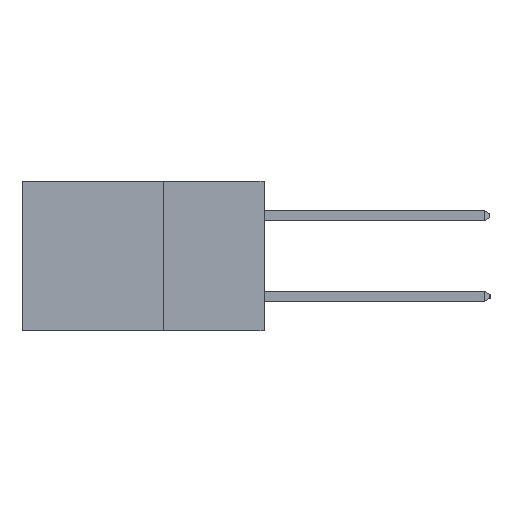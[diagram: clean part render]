
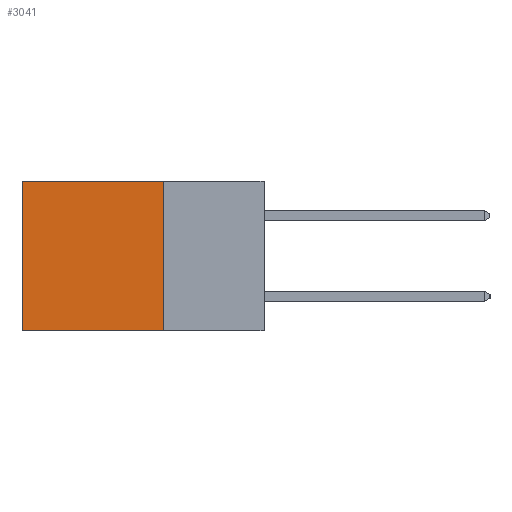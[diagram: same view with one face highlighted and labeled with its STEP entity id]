
A CAD part, left-side view. The second image highlights one B-rep face of the part: STEP entity #3041.
In plain terms, the highlighted planar face has unit normal (-1, 0, 0).
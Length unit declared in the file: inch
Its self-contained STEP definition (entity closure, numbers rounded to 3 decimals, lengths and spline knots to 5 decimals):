
#332 = ORIENTED_EDGE ( 'NONE', *, *, #6425, .F. ) ;
#567 = DIRECTION ( 'NONE',  ( 0., 1., 0. ) ) ;
#807 = CARTESIAN_POINT ( 'NONE',  ( 0.2615, 0.25, 0. ) ) ;
#886 = CARTESIAN_POINT ( 'NONE',  ( 0.2615, 0.25, -0.37 ) ) ;
#1542 = AXIS2_PLACEMENT_3D ( 'NONE', #5706, #8288, #3043 ) ;
#1579 = VERTEX_POINT ( 'NONE', #807 ) ;
#2264 = VERTEX_POINT ( 'NONE', #9968 ) ;
#2341 = VERTEX_POINT ( 'NONE', #3122 ) ;
#3041 = ADVANCED_FACE ( 'NONE', ( #8326 ), #9948, .F. ) ;
#3043 = DIRECTION ( 'NONE',  ( 0., 0., -1. ) ) ;
#3122 = CARTESIAN_POINT ( 'NONE',  ( 0.2615, 0.6, 0. ) ) ;
#3479 = ORIENTED_EDGE ( 'NONE', *, *, #8227, .T. ) ;
#3774 = EDGE_CURVE ( 'NONE', #1579, #10707, #7980, .T. ) ;
#3847 = VECTOR ( 'NONE', #7431, 39.37008 ) ;
#4026 = EDGE_CURVE ( 'NONE', #2341, #2264, #10570, .T. ) ;
#4866 = DIRECTION ( 'NONE',  ( 0., 0., -1. ) ) ;
#5706 = CARTESIAN_POINT ( 'NONE',  ( 0.2615, 0.25, -0.37 ) ) ;
#5800 = VECTOR ( 'NONE', #10179, 39.37008 ) ;
#6425 = EDGE_CURVE ( 'NONE', #10707, #2264, #11121, .T. ) ;
#6559 = CARTESIAN_POINT ( 'NONE',  ( 0.2615, 0.25, 0. ) ) ;
#6810 = CARTESIAN_POINT ( 'NONE',  ( 0.2615, 0.6, -0.37 ) ) ;
#6983 = VECTOR ( 'NONE', #567, 39.37008 ) ;
#7431 = DIRECTION ( 'NONE',  ( 0., 1., 0. ) ) ;
#7980 = LINE ( 'NONE', #886, #10199 ) ;
#8084 = CARTESIAN_POINT ( 'NONE',  ( 0.2615, 0.25, -0.37 ) ) ;
#8227 = EDGE_CURVE ( 'NONE', #1579, #2341, #10627, .T. ) ;
#8288 = DIRECTION ( 'NONE',  ( 1., 0., 0. ) ) ;
#8326 = FACE_OUTER_BOUND ( 'NONE', #10441, .T. ) ;
#9801 = ORIENTED_EDGE ( 'NONE', *, *, #4026, .T. ) ;
#9948 = PLANE ( 'NONE',  #1542 ) ;
#9968 = CARTESIAN_POINT ( 'NONE',  ( 0.2615, 0.6, -0.37 ) ) ;
#10071 = ORIENTED_EDGE ( 'NONE', *, *, #3774, .F. ) ;
#10179 = DIRECTION ( 'NONE',  ( 0., 0., -1. ) ) ;
#10199 = VECTOR ( 'NONE', #4866, 39.37008 ) ;
#10441 = EDGE_LOOP ( 'NONE', ( #9801, #332, #10071, #3479 ) ) ;
#10570 = LINE ( 'NONE', #6810, #5800 ) ;
#10627 = LINE ( 'NONE', #6559, #3847 ) ;
#10707 = VERTEX_POINT ( 'NONE', #8084 ) ;
#11121 = LINE ( 'NONE', #11288, #6983 ) ;
#11288 = CARTESIAN_POINT ( 'NONE',  ( 0.2615, 0.25, -0.37 ) ) ;
